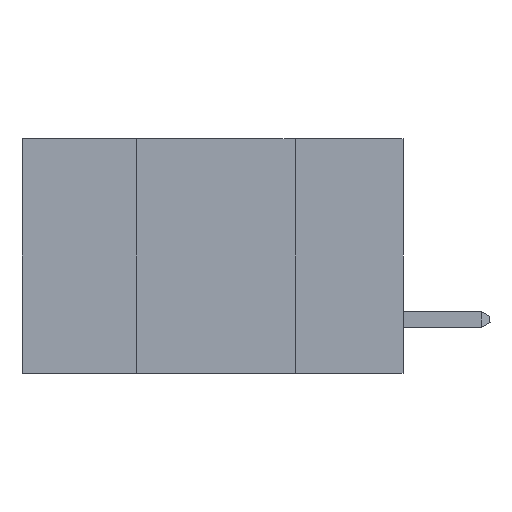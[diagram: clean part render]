
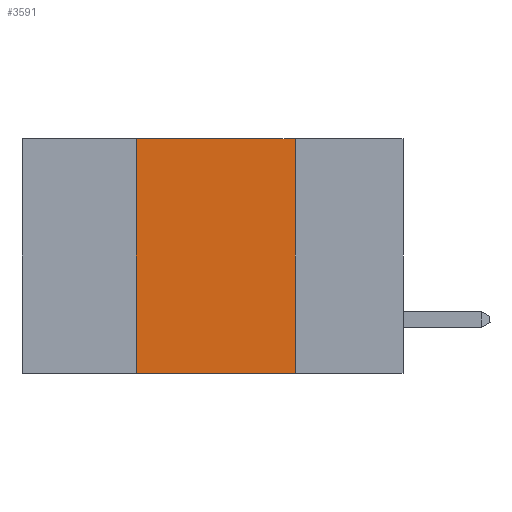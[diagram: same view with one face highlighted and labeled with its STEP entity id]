
A CAD part, left-side view. The second image highlights one B-rep face of the part: STEP entity #3591.
In plain terms, the highlighted planar face has unit normal (-1, 0, 0).
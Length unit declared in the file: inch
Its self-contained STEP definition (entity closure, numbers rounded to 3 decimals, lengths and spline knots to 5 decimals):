
#582 = CARTESIAN_POINT ( 'NONE',  ( 0., 0.42, -0.37 ) ) ;
#1297 = DIRECTION ( 'NONE',  ( 1., 0., 0. ) ) ;
#1409 = ORIENTED_EDGE ( 'NONE', *, *, #12740, .T. ) ;
#1445 = DIRECTION ( 'NONE',  ( 0., -1., 0. ) ) ;
#1849 = ORIENTED_EDGE ( 'NONE', *, *, #9525, .F. ) ;
#2525 = DIRECTION ( 'NONE',  ( 0., 0., -1. ) ) ;
#2920 = LINE ( 'NONE', #4279, #20725 ) ;
#3560 = CARTESIAN_POINT ( 'NONE',  ( 0., 0.6, 0. ) ) ;
#3591 = ADVANCED_FACE ( 'NONE', ( #9920 ), #21899, .F. ) ;
#4049 = VERTEX_POINT ( 'NONE', #12945 ) ;
#4279 = CARTESIAN_POINT ( 'NONE',  ( 0., 0.42, 0. ) ) ;
#6366 = LINE ( 'NONE', #13929, #13800 ) ;
#6726 = EDGE_LOOP ( 'NONE', ( #13269, #21263, #1849, #1409 ) ) ;
#8704 = CARTESIAN_POINT ( 'NONE',  ( 0., 0.17, 0. ) ) ;
#9525 = EDGE_CURVE ( 'NONE', #24717, #4049, #2920, .T. ) ;
#9658 = CARTESIAN_POINT ( 'NONE',  ( 0., 0.6, -0.37 ) ) ;
#9920 = FACE_OUTER_BOUND ( 'NONE', #6726, .T. ) ;
#10207 = CARTESIAN_POINT ( 'NONE',  ( 0., 0.17, -0.37 ) ) ;
#10560 = VERTEX_POINT ( 'NONE', #8704 ) ;
#11075 = EDGE_CURVE ( 'NONE', #10560, #14523, #14427, .T. ) ;
#11777 = DIRECTION ( 'NONE',  ( 0., 0., -1. ) ) ;
#12740 = EDGE_CURVE ( 'NONE', #24717, #14523, #23733, .T. ) ;
#12945 = CARTESIAN_POINT ( 'NONE',  ( 0., 0.42, 0. ) ) ;
#13269 = ORIENTED_EDGE ( 'NONE', *, *, #11075, .F. ) ;
#13691 = VECTOR ( 'NONE', #1445, 39.37008 ) ;
#13800 = VECTOR ( 'NONE', #26805, 39.37008 ) ;
#13929 = CARTESIAN_POINT ( 'NONE',  ( 0., 0.6, 0. ) ) ;
#14427 = LINE ( 'NONE', #20978, #20880 ) ;
#14523 = VERTEX_POINT ( 'NONE', #10207 ) ;
#20725 = VECTOR ( 'NONE', #22730, 39.37008 ) ;
#20880 = VECTOR ( 'NONE', #2525, 39.37008 ) ;
#20978 = CARTESIAN_POINT ( 'NONE',  ( 0., 0.17, 0. ) ) ;
#21263 = ORIENTED_EDGE ( 'NONE', *, *, #23201, .F. ) ;
#21899 = PLANE ( 'NONE',  #23849 ) ;
#22730 = DIRECTION ( 'NONE',  ( 0., 0., 1. ) ) ;
#23201 = EDGE_CURVE ( 'NONE', #4049, #10560, #6366, .T. ) ;
#23733 = LINE ( 'NONE', #9658, #13691 ) ;
#23849 = AXIS2_PLACEMENT_3D ( 'NONE', #3560, #1297, #11777 ) ;
#24717 = VERTEX_POINT ( 'NONE', #582 ) ;
#26805 = DIRECTION ( 'NONE',  ( 0., -1., 0. ) ) ;
